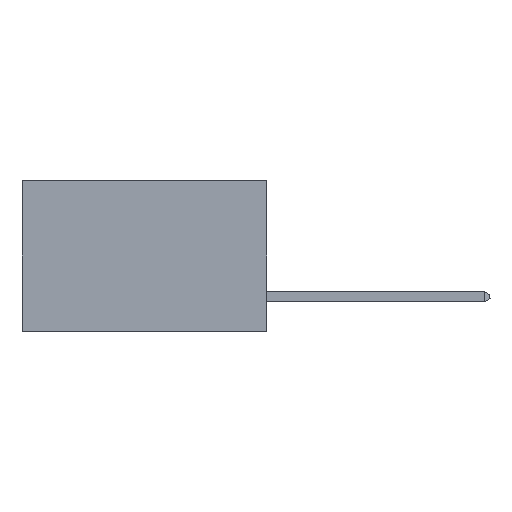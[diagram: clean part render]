
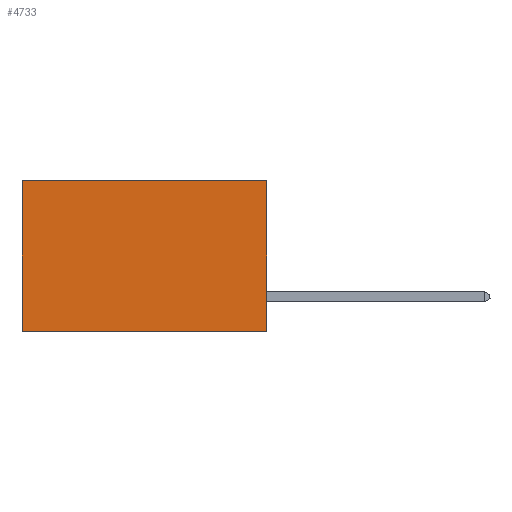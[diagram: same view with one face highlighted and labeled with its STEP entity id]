
A CAD part, left-side view. The second image highlights one B-rep face of the part: STEP entity #4733.
In plain terms, the highlighted planar face has unit normal (-1, 0, 0).
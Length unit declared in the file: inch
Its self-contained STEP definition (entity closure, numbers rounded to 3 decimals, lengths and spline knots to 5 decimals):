
#40 = VECTOR ( 'NONE', #10616, 39.37008 ) ;
#371 = CARTESIAN_POINT ( 'NONE',  ( 0.2875, 0.6, 0. ) ) ;
#629 = CARTESIAN_POINT ( 'NONE',  ( 0.2875, 0., 0. ) ) ;
#1361 = EDGE_CURVE ( 'NONE', #8910, #8914, #9340, .T. ) ;
#1395 = VECTOR ( 'NONE', #10190, 39.37008 ) ;
#3863 = LINE ( 'NONE', #12396, #1395 ) ;
#4186 = EDGE_LOOP ( 'NONE', ( #4219, #5118, #8692, #5694 ) ) ;
#4219 = ORIENTED_EDGE ( 'NONE', *, *, #1361, .T. ) ;
#4333 = CARTESIAN_POINT ( 'NONE',  ( 0.2875, 0., 0. ) ) ;
#4733 = ADVANCED_FACE ( 'NONE', ( #9228 ), #4776, .F. ) ;
#4776 = PLANE ( 'NONE',  #5762 ) ;
#4880 = CARTESIAN_POINT ( 'NONE',  ( 0.2875, 0., 0. ) ) ;
#5118 = ORIENTED_EDGE ( 'NONE', *, *, #10501, .F. ) ;
#5180 = LINE ( 'NONE', #629, #40 ) ;
#5694 = ORIENTED_EDGE ( 'NONE', *, *, #8789, .T. ) ;
#5762 = AXIS2_PLACEMENT_3D ( 'NONE', #4880, #9357, #13931 ) ;
#7011 = DIRECTION ( 'NONE',  ( 0., 1., 0. ) ) ;
#7695 = VECTOR ( 'NONE', #7011, 39.37008 ) ;
#8121 = VECTOR ( 'NONE', #10316, 39.37008 ) ;
#8692 = ORIENTED_EDGE ( 'NONE', *, *, #11970, .F. ) ;
#8789 = EDGE_CURVE ( 'NONE', #12309, #8910, #3863, .T. ) ;
#8910 = VERTEX_POINT ( 'NONE', #371 ) ;
#8914 = VERTEX_POINT ( 'NONE', #13932 ) ;
#9014 = VERTEX_POINT ( 'NONE', #10941 ) ;
#9228 = FACE_OUTER_BOUND ( 'NONE', #4186, .T. ) ;
#9340 = LINE ( 'NONE', #13373, #8121 ) ;
#9357 = DIRECTION ( 'NONE',  ( 1., 0., 0. ) ) ;
#10190 = DIRECTION ( 'NONE',  ( 0., 1., 0. ) ) ;
#10316 = DIRECTION ( 'NONE',  ( 0., 0., -1. ) ) ;
#10501 = EDGE_CURVE ( 'NONE', #9014, #8914, #10847, .T. ) ;
#10616 = DIRECTION ( 'NONE',  ( 0., 0., -1. ) ) ;
#10847 = LINE ( 'NONE', #11485, #7695 ) ;
#10941 = CARTESIAN_POINT ( 'NONE',  ( 0.2875, 0., -0.37 ) ) ;
#11485 = CARTESIAN_POINT ( 'NONE',  ( 0.2875, 0., -0.37 ) ) ;
#11970 = EDGE_CURVE ( 'NONE', #12309, #9014, #5180, .T. ) ;
#12309 = VERTEX_POINT ( 'NONE', #4333 ) ;
#12396 = CARTESIAN_POINT ( 'NONE',  ( 0.2875, 0., 0. ) ) ;
#13373 = CARTESIAN_POINT ( 'NONE',  ( 0.2875, 0.6, 0. ) ) ;
#13931 = DIRECTION ( 'NONE',  ( 0., 0., -1. ) ) ;
#13932 = CARTESIAN_POINT ( 'NONE',  ( 0.2875, 0.6, -0.37 ) ) ;
